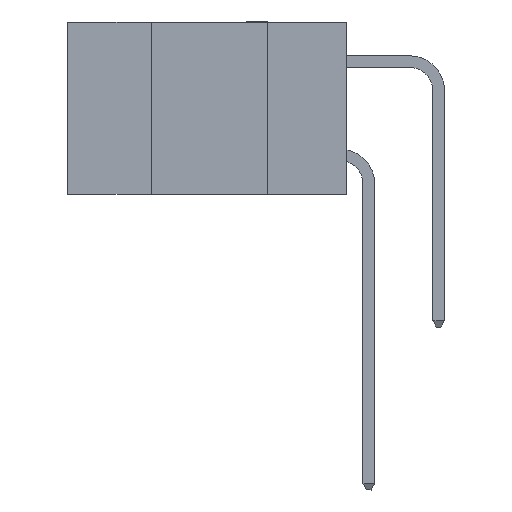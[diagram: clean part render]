
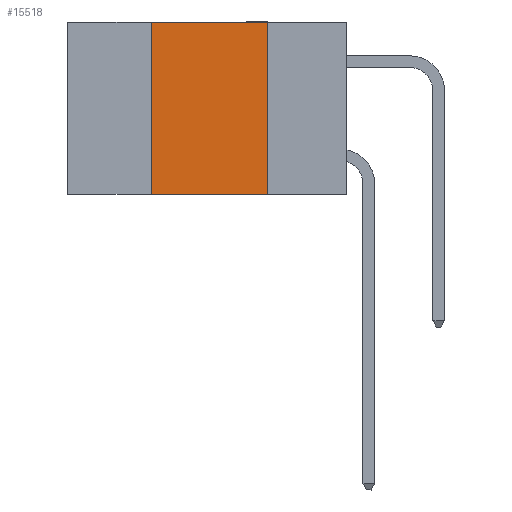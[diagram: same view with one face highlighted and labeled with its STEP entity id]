
A CAD part, left-side view. The second image highlights one B-rep face of the part: STEP entity #15518.
In plain terms, the highlighted planar face has unit normal (-1, 0, 0).
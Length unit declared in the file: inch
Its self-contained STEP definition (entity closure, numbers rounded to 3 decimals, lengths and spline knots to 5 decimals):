
#199 = VECTOR ( 'NONE', #10236, 39.37008 ) ;
#2236 = PLANE ( 'NONE',  #16435 ) ;
#2438 = EDGE_LOOP ( 'NONE', ( #3159, #17557, #8614, #13389 ) ) ;
#2781 = EDGE_CURVE ( 'NONE', #13726, #12153, #12087, .T. ) ;
#2805 = LINE ( 'NONE', #14270, #8445 ) ;
#2904 = CARTESIAN_POINT ( 'NONE',  ( 0., 0.6, 0. ) ) ;
#3159 = ORIENTED_EDGE ( 'NONE', *, *, #7210, .F. ) ;
#3475 = CARTESIAN_POINT ( 'NONE',  ( 0., 0.42, -0.37 ) ) ;
#4522 = DIRECTION ( 'NONE',  ( 0., 0., -1. ) ) ;
#5994 = CARTESIAN_POINT ( 'NONE',  ( 0., 0.17, 0. ) ) ;
#7076 = DIRECTION ( 'NONE',  ( 0., 0., 1. ) ) ;
#7210 = EDGE_CURVE ( 'NONE', #8128, #12153, #11360, .T. ) ;
#8052 = VERTEX_POINT ( 'NONE', #15110 ) ;
#8128 = VERTEX_POINT ( 'NONE', #12697 ) ;
#8445 = VECTOR ( 'NONE', #7076, 39.37008 ) ;
#8526 = CARTESIAN_POINT ( 'NONE',  ( 0., 0.17, -0.37 ) ) ;
#8614 = ORIENTED_EDGE ( 'NONE', *, *, #13976, .F. ) ;
#10048 = LINE ( 'NONE', #2904, #199 ) ;
#10236 = DIRECTION ( 'NONE',  ( 0., -1., 0. ) ) ;
#10860 = VECTOR ( 'NONE', #13390, 39.37008 ) ;
#11319 = VECTOR ( 'NONE', #4522, 39.37008 ) ;
#11360 = LINE ( 'NONE', #5994, #11319 ) ;
#12087 = LINE ( 'NONE', #13213, #10860 ) ;
#12153 = VERTEX_POINT ( 'NONE', #8526 ) ;
#12697 = CARTESIAN_POINT ( 'NONE',  ( 0., 0.17, 0. ) ) ;
#13213 = CARTESIAN_POINT ( 'NONE',  ( 0., 0.6, -0.37 ) ) ;
#13389 = ORIENTED_EDGE ( 'NONE', *, *, #2781, .T. ) ;
#13390 = DIRECTION ( 'NONE',  ( 0., -1., 0. ) ) ;
#13726 = VERTEX_POINT ( 'NONE', #3475 ) ;
#13976 = EDGE_CURVE ( 'NONE', #13726, #8052, #2805, .T. ) ;
#14270 = CARTESIAN_POINT ( 'NONE',  ( 0., 0.42, 0. ) ) ;
#15110 = CARTESIAN_POINT ( 'NONE',  ( 0., 0.42, 0. ) ) ;
#15233 = EDGE_CURVE ( 'NONE', #8052, #8128, #10048, .T. ) ;
#15273 = DIRECTION ( 'NONE',  ( 0., 0., -1. ) ) ;
#15518 = ADVANCED_FACE ( 'NONE', ( #16745 ), #2236, .F. ) ;
#16383 = CARTESIAN_POINT ( 'NONE',  ( 0., 0.6, 0. ) ) ;
#16435 = AXIS2_PLACEMENT_3D ( 'NONE', #16383, #17864, #15273 ) ;
#16745 = FACE_OUTER_BOUND ( 'NONE', #2438, .T. ) ;
#17557 = ORIENTED_EDGE ( 'NONE', *, *, #15233, .F. ) ;
#17864 = DIRECTION ( 'NONE',  ( 1., 0., 0. ) ) ;
